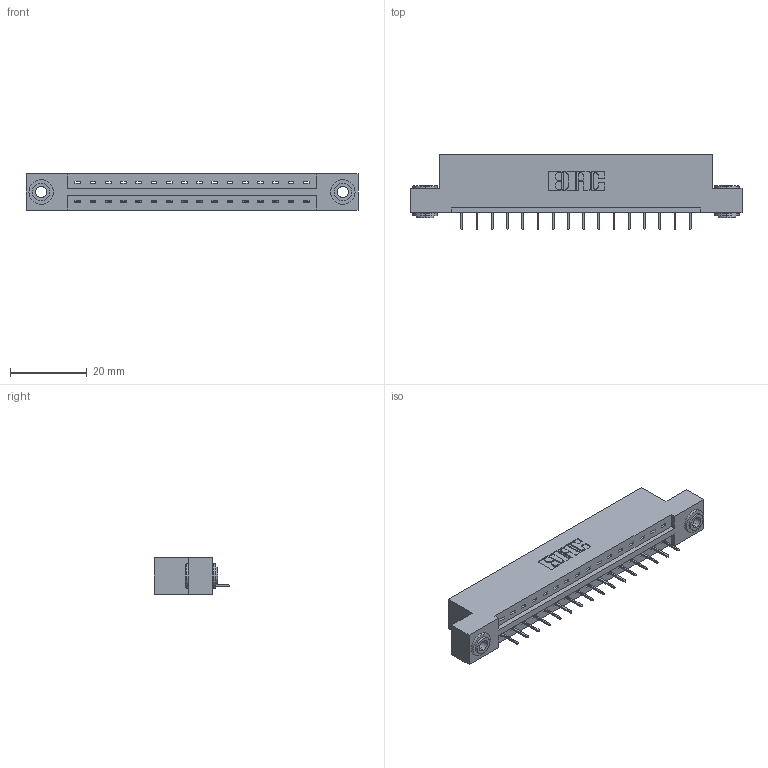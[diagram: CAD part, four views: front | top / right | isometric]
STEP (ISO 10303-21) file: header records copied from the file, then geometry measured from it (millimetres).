
FILE_DESCRIPTION (( 'STEP AP203' ), '1' );
FILE_NAME ('337-016-524-103.STEP', '2019-09-28T17:34:44', ( '' ), ( '' ), 'SwSTEP 2.0', 'SolidWorks 2016', '' );
FILE_SCHEMA (( 'CONFIG_CONTROL_DESIGN' ));
Length unit declared in the file: inch
Products named in the file (4): 345-250-002_345-250-002-102; 345-292-001_345-293-124; 337 Part_Flush Mounting Lugs - 0.156 Dia-TH; 337-016-524-103
Assembly tree (19 placements, depth 2):
  337-016-524-103
    337 Part_Flush Mounting Lugs - 0.156 Dia-TH
    345-292-001_345-293-124  x16
    345-250-002_345-250-002-102  x2
Bounding box: 86.41 x 19.69 x 9.4 mm (x, y, z)
Volume: 8611.8 mm3; surface area: 8765.1 mm2
Topology: 19 solids, 19 shells, 1208 faces, 3459 edges, 2238 vertices
Faces by surface type: plane 912, cylinder 288, cone 8
Entity records: 15980 total; most frequent: CARTESIAN_POINT 2757, ORIENTED_EDGE 2702, DIRECTION 2409, EDGE_CURVE 1351, LINE 1203, VECTOR 1203, VERTEX_POINT 894, AXIS2_PLACEMENT_3D 603
